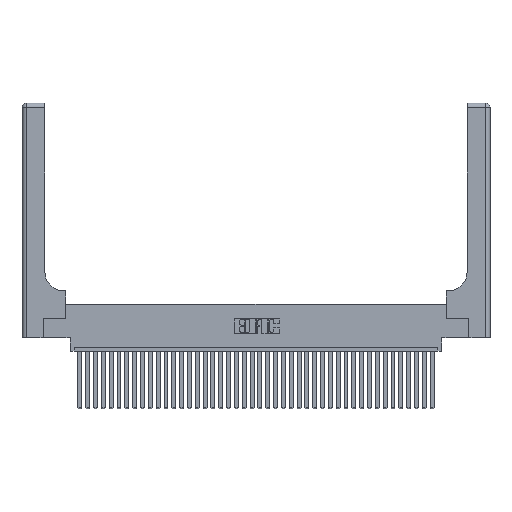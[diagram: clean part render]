
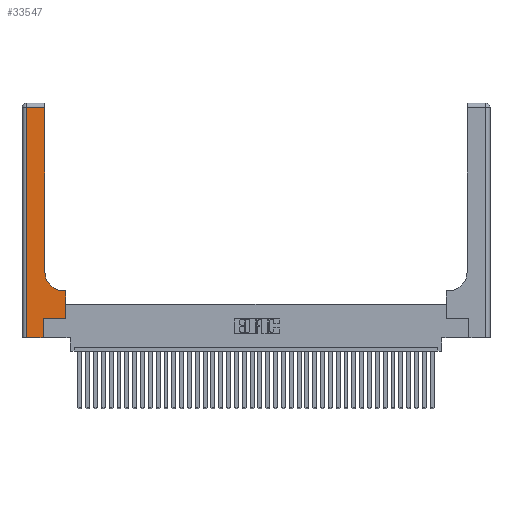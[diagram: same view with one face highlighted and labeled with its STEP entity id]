
A CAD part, top view. The second image highlights one B-rep face of the part: STEP entity #33547.
In plain terms, the highlighted planar face has unit normal (0, 0, 1).
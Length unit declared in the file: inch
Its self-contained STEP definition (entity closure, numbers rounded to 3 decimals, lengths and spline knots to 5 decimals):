
#1056 = DIRECTION ( 'NONE',  ( 1., 0., 0. ) ) ;
#1124 = DIRECTION ( 'NONE',  ( -1., 0., 0. ) ) ;
#1142 = VECTOR ( 'NONE', #13467, 39.37008 ) ;
#1761 = CIRCLE ( 'NONE', #10734, 0.25 ) ;
#2010 = DIRECTION ( 'NONE',  ( -1., 0., 0. ) ) ;
#2662 = VECTOR ( 'NONE', #21859, 39.37008 ) ;
#2724 = VECTOR ( 'NONE', #2010, 39.37008 ) ;
#3337 = DIRECTION ( 'NONE',  ( -1., 0., 0. ) ) ;
#3622 = LINE ( 'NONE', #29086, #2724 ) ;
#4012 = LINE ( 'NONE', #31645, #1142 ) ;
#4217 = LINE ( 'NONE', #14061, #19406 ) ;
#5018 = ORIENTED_EDGE ( 'NONE', *, *, #22760, .T. ) ;
#5110 = VERTEX_POINT ( 'NONE', #32292 ) ;
#5129 = CARTESIAN_POINT ( 'NONE',  ( 0.06, 3., 0.37 ) ) ;
#5282 = CARTESIAN_POINT ( 'NONE',  ( 0.5415, 0.6, 0.37 ) ) ;
#5422 = CARTESIAN_POINT ( 'NONE',  ( 0.269, 0.25, 0.37 ) ) ;
#5535 = EDGE_CURVE ( 'NONE', #9735, #21779, #16546, .T. ) ;
#5738 = CARTESIAN_POINT ( 'NONE',  ( 0.2915, 2.94, 0.37 ) ) ;
#6778 = LINE ( 'NONE', #25195, #28616 ) ;
#7958 = AXIS2_PLACEMENT_3D ( 'NONE', #25389, #22636, #1124 ) ;
#8612 = LINE ( 'NONE', #24428, #9069 ) ;
#9069 = VECTOR ( 'NONE', #3337, 39.37008 ) ;
#9735 = VERTEX_POINT ( 'NONE', #29394 ) ;
#9923 = CARTESIAN_POINT ( 'NONE',  ( 0., 0., 0.37 ) ) ;
#10734 = AXIS2_PLACEMENT_3D ( 'NONE', #16876, #11281, #20446 ) ;
#10839 = VECTOR ( 'NONE', #28866, 39.37008 ) ;
#11138 = VERTEX_POINT ( 'NONE', #5422 ) ;
#11281 = DIRECTION ( 'NONE',  ( 0., 0., -1. ) ) ;
#11968 = CARTESIAN_POINT ( 'NONE',  ( 0.06, 0., 0.37 ) ) ;
#12550 = EDGE_CURVE ( 'NONE', #38608, #14880, #4217, .T. ) ;
#12677 = FACE_OUTER_BOUND ( 'NONE', #36903, .T. ) ;
#13447 = EDGE_CURVE ( 'NONE', #21779, #20277, #3622, .T. ) ;
#13467 = DIRECTION ( 'NONE',  ( 0., 1., 0. ) ) ;
#14061 = CARTESIAN_POINT ( 'NONE',  ( 0.5585, 0.25, 0.37 ) ) ;
#14880 = VERTEX_POINT ( 'NONE', #25175 ) ;
#15108 = LINE ( 'NONE', #5129, #10839 ) ;
#15366 = ORIENTED_EDGE ( 'NONE', *, *, #13447, .T. ) ;
#15512 = VERTEX_POINT ( 'NONE', #11968 ) ;
#15560 = VECTOR ( 'NONE', #35385, 39.37008 ) ;
#16546 = LINE ( 'NONE', #22822, #15560 ) ;
#16876 = CARTESIAN_POINT ( 'NONE',  ( 0.5415, 0.85, 0.37 ) ) ;
#19185 = ORIENTED_EDGE ( 'NONE', *, *, #5535, .T. ) ;
#19406 = VECTOR ( 'NONE', #35259, 39.37008 ) ;
#20277 = VERTEX_POINT ( 'NONE', #21567 ) ;
#20446 = DIRECTION ( 'NONE',  ( 1., 0., 0. ) ) ;
#21567 = CARTESIAN_POINT ( 'NONE',  ( 0.06, 2.94, 0.37 ) ) ;
#21779 = VERTEX_POINT ( 'NONE', #5738 ) ;
#21859 = DIRECTION ( 'NONE',  ( 1., 0., 0. ) ) ;
#21920 = ORIENTED_EDGE ( 'NONE', *, *, #35563, .T. ) ;
#22636 = DIRECTION ( 'NONE',  ( 0., 0., -1. ) ) ;
#22760 = EDGE_CURVE ( 'NONE', #32954, #9735, #1761, .T. ) ;
#22770 = PLANE ( 'NONE',  #7958 ) ;
#22778 = ORIENTED_EDGE ( 'NONE', *, *, #30245, .T. ) ;
#22822 = CARTESIAN_POINT ( 'NONE',  ( 0.2915, 3., 0.37 ) ) ;
#24428 = CARTESIAN_POINT ( 'NONE',  ( 0.2915, 0.6, 0.37 ) ) ;
#25175 = CARTESIAN_POINT ( 'NONE',  ( 0.5585, 0.6, 0.37 ) ) ;
#25195 = CARTESIAN_POINT ( 'NONE',  ( 0.269, 0.25, 0.37 ) ) ;
#25389 = CARTESIAN_POINT ( 'NONE',  ( 0., 3., 0.37 ) ) ;
#27200 = CARTESIAN_POINT ( 'NONE',  ( 0.5585, 0.25, 0.37 ) ) ;
#28616 = VECTOR ( 'NONE', #1056, 39.37008 ) ;
#28866 = DIRECTION ( 'NONE',  ( 0., -1., 0. ) ) ;
#29086 = CARTESIAN_POINT ( 'NONE',  ( 0., 2.94, 0.37 ) ) ;
#29394 = CARTESIAN_POINT ( 'NONE',  ( 0.2915, 0.85, 0.37 ) ) ;
#29563 = ORIENTED_EDGE ( 'NONE', *, *, #38701, .T. ) ;
#30245 = EDGE_CURVE ( 'NONE', #11138, #38608, #6778, .T. ) ;
#30361 = ORIENTED_EDGE ( 'NONE', *, *, #35459, .T. ) ;
#30920 = ORIENTED_EDGE ( 'NONE', *, *, #12550, .T. ) ;
#31598 = LINE ( 'NONE', #9923, #2662 ) ;
#31645 = CARTESIAN_POINT ( 'NONE',  ( 0.269, 0., 0.37 ) ) ;
#32224 = ORIENTED_EDGE ( 'NONE', *, *, #35799, .T. ) ;
#32292 = CARTESIAN_POINT ( 'NONE',  ( 0.269, 0., 0.37 ) ) ;
#32954 = VERTEX_POINT ( 'NONE', #5282 ) ;
#33547 = ADVANCED_FACE ( 'NONE', ( #12677 ), #22770, .F. ) ;
#35259 = DIRECTION ( 'NONE',  ( 0., 1., 0. ) ) ;
#35385 = DIRECTION ( 'NONE',  ( 0., 1., 0. ) ) ;
#35459 = EDGE_CURVE ( 'NONE', #5110, #11138, #4012, .T. ) ;
#35563 = EDGE_CURVE ( 'NONE', #20277, #15512, #15108, .T. ) ;
#35799 = EDGE_CURVE ( 'NONE', #14880, #32954, #8612, .T. ) ;
#36903 = EDGE_LOOP ( 'NONE', ( #19185, #15366, #21920, #29563, #30361, #22778, #30920, #32224, #5018 ) ) ;
#38608 = VERTEX_POINT ( 'NONE', #27200 ) ;
#38701 = EDGE_CURVE ( 'NONE', #15512, #5110, #31598, .T. ) ;
